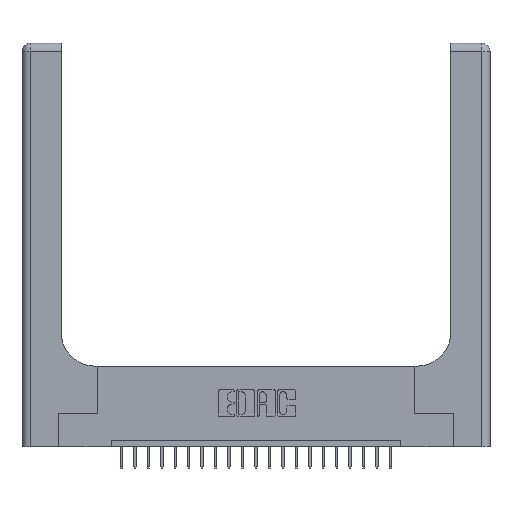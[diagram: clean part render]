
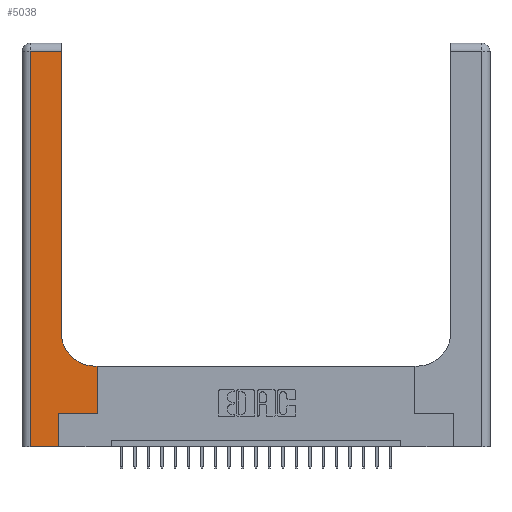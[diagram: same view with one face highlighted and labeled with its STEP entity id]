
A CAD part, top view. The second image highlights one B-rep face of the part: STEP entity #5038.
In plain terms, the highlighted planar face has unit normal (0, 0, 1).
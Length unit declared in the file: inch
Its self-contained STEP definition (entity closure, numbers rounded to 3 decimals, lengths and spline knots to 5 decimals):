
#114 = LINE ( 'NONE', #3668, #14496 ) ;
#232 = CARTESIAN_POINT ( 'NONE',  ( 0.2915, 0.6, 0.37 ) ) ;
#248 = DIRECTION ( 'NONE',  ( 1., 0., 0. ) ) ;
#473 = VECTOR ( 'NONE', #13484, 39.37008 ) ;
#499 = ORIENTED_EDGE ( 'NONE', *, *, #21401, .T. ) ;
#1245 = CARTESIAN_POINT ( 'NONE',  ( 0., 3., 0.37 ) ) ;
#1718 = CIRCLE ( 'NONE', #15015, 0.25 ) ;
#1742 = ORIENTED_EDGE ( 'NONE', *, *, #21307, .T. ) ;
#1746 = EDGE_LOOP ( 'NONE', ( #10841, #13161, #18229, #2375, #21656, #9336, #499, #1742, #20736 ) ) ;
#1921 = LINE ( 'NONE', #2828, #20935 ) ;
#2375 = ORIENTED_EDGE ( 'NONE', *, *, #22485, .T. ) ;
#2609 = CARTESIAN_POINT ( 'NONE',  ( 0.2915, 3., 0.37 ) ) ;
#2828 = CARTESIAN_POINT ( 'NONE',  ( 0.5585, 0.25, 0.37 ) ) ;
#2905 = DIRECTION ( 'NONE',  ( 0., 1., 0. ) ) ;
#3372 = LINE ( 'NONE', #7952, #473 ) ;
#3558 = AXIS2_PLACEMENT_3D ( 'NONE', #1245, #23494, #8543 ) ;
#3668 = CARTESIAN_POINT ( 'NONE',  ( 0., 0., 0.37 ) ) ;
#4991 = CARTESIAN_POINT ( 'NONE',  ( 0.2915, 2.94, 0.37 ) ) ;
#5038 = ADVANCED_FACE ( 'NONE', ( #12332 ), #8789, .F. ) ;
#5189 = DIRECTION ( 'NONE',  ( 0., 0., -1. ) ) ;
#5618 = CARTESIAN_POINT ( 'NONE',  ( 0.06, 2.94, 0.37 ) ) ;
#5654 = CARTESIAN_POINT ( 'NONE',  ( 0.269, 0., 0.37 ) ) ;
#6086 = LINE ( 'NONE', #21885, #20162 ) ;
#7274 = DIRECTION ( 'NONE',  ( -1., 0., 0. ) ) ;
#7553 = DIRECTION ( 'NONE',  ( 0., 1., 0. ) ) ;
#7952 = CARTESIAN_POINT ( 'NONE',  ( 0.269, 0.25, 0.37 ) ) ;
#8453 = EDGE_CURVE ( 'NONE', #22971, #21681, #22912, .T. ) ;
#8509 = VECTOR ( 'NONE', #11350, 39.37008 ) ;
#8524 = VERTEX_POINT ( 'NONE', #11977 ) ;
#8543 = DIRECTION ( 'NONE',  ( -1., 0., 0. ) ) ;
#8789 = PLANE ( 'NONE',  #3558 ) ;
#9221 = CARTESIAN_POINT ( 'NONE',  ( 0.269, 0., 0.37 ) ) ;
#9336 = ORIENTED_EDGE ( 'NONE', *, *, #21358, .T. ) ;
#9650 = VERTEX_POINT ( 'NONE', #14424 ) ;
#10841 = ORIENTED_EDGE ( 'NONE', *, *, #11921, .T. ) ;
#10885 = CARTESIAN_POINT ( 'NONE',  ( 0.2915, 0.85, 0.37 ) ) ;
#11350 = DIRECTION ( 'NONE',  ( -1., 0., 0. ) ) ;
#11652 = VERTEX_POINT ( 'NONE', #10885 ) ;
#11686 = EDGE_CURVE ( 'NONE', #22737, #20571, #6086, .T. ) ;
#11696 = LINE ( 'NONE', #232, #8509 ) ;
#11921 = EDGE_CURVE ( 'NONE', #11652, #22737, #15812, .T. ) ;
#11977 = CARTESIAN_POINT ( 'NONE',  ( 0.5585, 0.6, 0.37 ) ) ;
#12015 = CARTESIAN_POINT ( 'NONE',  ( 0.06, 0., 0.37 ) ) ;
#12039 = EDGE_CURVE ( 'NONE', #12879, #11652, #1718, .T. ) ;
#12332 = FACE_OUTER_BOUND ( 'NONE', #1746, .T. ) ;
#12879 = VERTEX_POINT ( 'NONE', #22714 ) ;
#12920 = CARTESIAN_POINT ( 'NONE',  ( 0.269, 0.25, 0.37 ) ) ;
#13161 = ORIENTED_EDGE ( 'NONE', *, *, #11686, .T. ) ;
#13484 = DIRECTION ( 'NONE',  ( 1., 0., 0. ) ) ;
#13501 = VECTOR ( 'NONE', #19163, 39.37008 ) ;
#14028 = CARTESIAN_POINT ( 'NONE',  ( 0.5415, 0.85, 0.37 ) ) ;
#14424 = CARTESIAN_POINT ( 'NONE',  ( 0.5585, 0.25, 0.37 ) ) ;
#14496 = VECTOR ( 'NONE', #248, 39.37008 ) ;
#14511 = VECTOR ( 'NONE', #7553, 39.37008 ) ;
#15015 = AXIS2_PLACEMENT_3D ( 'NONE', #14028, #5189, #23084 ) ;
#15812 = LINE ( 'NONE', #2609, #13501 ) ;
#16938 = VECTOR ( 'NONE', #17626, 39.37008 ) ;
#17588 = VERTEX_POINT ( 'NONE', #12015 ) ;
#17626 = DIRECTION ( 'NONE',  ( 0., -1., 0. ) ) ;
#18229 = ORIENTED_EDGE ( 'NONE', *, *, #20794, .T. ) ;
#18935 = LINE ( 'NONE', #23144, #16938 ) ;
#19163 = DIRECTION ( 'NONE',  ( 0., 1., 0. ) ) ;
#20162 = VECTOR ( 'NONE', #7274, 39.37008 ) ;
#20571 = VERTEX_POINT ( 'NONE', #5618 ) ;
#20736 = ORIENTED_EDGE ( 'NONE', *, *, #12039, .T. ) ;
#20794 = EDGE_CURVE ( 'NONE', #20571, #17588, #18935, .T. ) ;
#20935 = VECTOR ( 'NONE', #2905, 39.37008 ) ;
#21307 = EDGE_CURVE ( 'NONE', #8524, #12879, #11696, .T. ) ;
#21358 = EDGE_CURVE ( 'NONE', #21681, #9650, #3372, .T. ) ;
#21401 = EDGE_CURVE ( 'NONE', #9650, #8524, #1921, .T. ) ;
#21656 = ORIENTED_EDGE ( 'NONE', *, *, #8453, .T. ) ;
#21681 = VERTEX_POINT ( 'NONE', #12920 ) ;
#21885 = CARTESIAN_POINT ( 'NONE',  ( 0., 2.94, 0.37 ) ) ;
#22485 = EDGE_CURVE ( 'NONE', #17588, #22971, #114, .T. ) ;
#22714 = CARTESIAN_POINT ( 'NONE',  ( 0.5415, 0.6, 0.37 ) ) ;
#22737 = VERTEX_POINT ( 'NONE', #4991 ) ;
#22912 = LINE ( 'NONE', #9221, #14511 ) ;
#22971 = VERTEX_POINT ( 'NONE', #5654 ) ;
#23084 = DIRECTION ( 'NONE',  ( 1., 0., 0. ) ) ;
#23144 = CARTESIAN_POINT ( 'NONE',  ( 0.06, 3., 0.37 ) ) ;
#23494 = DIRECTION ( 'NONE',  ( 0., 0., -1. ) ) ;
